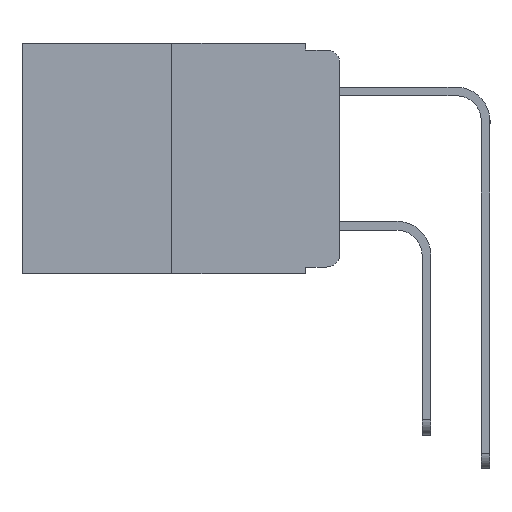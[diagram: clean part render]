
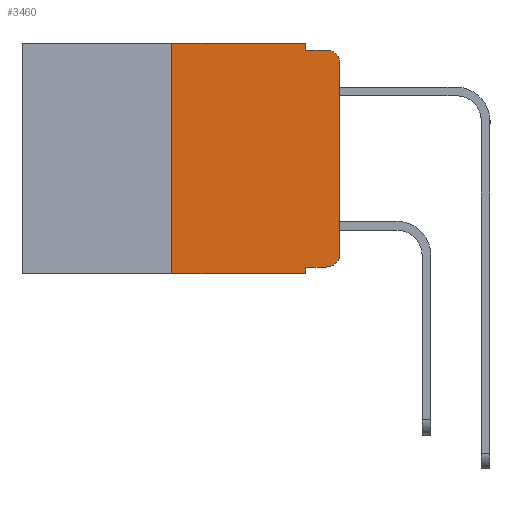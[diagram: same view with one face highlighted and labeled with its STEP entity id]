
A CAD part, left-side view. The second image highlights one B-rep face of the part: STEP entity #3460.
In plain terms, the highlighted planar face has unit normal (-1, 0, 0).
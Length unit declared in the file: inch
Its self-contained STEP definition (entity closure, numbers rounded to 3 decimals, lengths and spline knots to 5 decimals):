
#546 = VERTEX_POINT ( 'NONE', #12753 ) ;
#858 = CARTESIAN_POINT ( 'NONE',  ( 0., 0.02, -0.01 ) ) ;
#982 = ORIENTED_EDGE ( 'NONE', *, *, #9018, .F. ) ;
#1259 = VERTEX_POINT ( 'NONE', #13087 ) ;
#1698 = VERTEX_POINT ( 'NONE', #11523 ) ;
#2021 = PLANE ( 'NONE',  #4826 ) ;
#2198 = VERTEX_POINT ( 'NONE', #6630 ) ;
#2219 = DIRECTION ( 'NONE',  ( -1., 0., 0. ) ) ;
#2430 = VECTOR ( 'NONE', #13851, 39.37008 ) ;
#2683 = DIRECTION ( 'NONE',  ( 0., 0., 1. ) ) ;
#2816 = LINE ( 'NONE', #3233, #8758 ) ;
#3087 = CARTESIAN_POINT ( 'NONE',  ( 0., 0.473, 0. ) ) ;
#3233 = CARTESIAN_POINT ( 'NONE',  ( 0., 0.051, 0. ) ) ;
#3365 = CARTESIAN_POINT ( 'NONE',  ( 0., 0.051, 0. ) ) ;
#3460 = ADVANCED_FACE ( 'NONE', ( #4132 ), #2021, .F. ) ;
#3507 = VERTEX_POINT ( 'NONE', #858 ) ;
#3529 = VERTEX_POINT ( 'NONE', #14933 ) ;
#4132 = FACE_OUTER_BOUND ( 'NONE', #9407, .T. ) ;
#4143 = CIRCLE ( 'NONE', #9887, 0.02 ) ;
#4309 = DIRECTION ( 'NONE',  ( 0., -1., 0. ) ) ;
#4321 = VECTOR ( 'NONE', #9807, 39.37008 ) ;
#4395 = CARTESIAN_POINT ( 'NONE',  ( 0., 0.473, -0.343 ) ) ;
#4448 = DIRECTION ( 'NONE',  ( 1., 0., 0. ) ) ;
#4803 = EDGE_CURVE ( 'NONE', #1698, #1259, #10125, .T. ) ;
#4826 = AXIS2_PLACEMENT_3D ( 'NONE', #11409, #4448, #12557 ) ;
#5073 = CARTESIAN_POINT ( 'NONE',  ( 0., 0., 0. ) ) ;
#5165 = LINE ( 'NONE', #7351, #14039 ) ;
#5245 = ORIENTED_EDGE ( 'NONE', *, *, #7801, .T. ) ;
#5293 = DIRECTION ( 'NONE',  ( -1., 0., 0. ) ) ;
#5328 = ORIENTED_EDGE ( 'NONE', *, *, #4803, .F. ) ;
#5594 = VERTEX_POINT ( 'NONE', #12697 ) ;
#5635 = CARTESIAN_POINT ( 'NONE',  ( 0., 0.051, -0.01 ) ) ;
#6004 = ORIENTED_EDGE ( 'NONE', *, *, #7669, .F. ) ;
#6391 = CIRCLE ( 'NONE', #9435, 0.02 ) ;
#6630 = CARTESIAN_POINT ( 'NONE',  ( 0., 0.051, -0.333 ) ) ;
#6876 = ORIENTED_EDGE ( 'NONE', *, *, #14303, .F. ) ;
#6917 = VERTEX_POINT ( 'NONE', #13017 ) ;
#6990 = VECTOR ( 'NONE', #9794, 39.37008 ) ;
#7351 = CARTESIAN_POINT ( 'NONE',  ( 0., 0.25, 0. ) ) ;
#7669 = EDGE_CURVE ( 'NONE', #1259, #12660, #2816, .T. ) ;
#7801 = EDGE_CURVE ( 'NONE', #6917, #3529, #4143, .T. ) ;
#7950 = DIRECTION ( 'NONE',  ( 0., 0., -1. ) ) ;
#8338 = LINE ( 'NONE', #5635, #9075 ) ;
#8619 = CARTESIAN_POINT ( 'NONE',  ( 0., 0.051, -0.333 ) ) ;
#8758 = VECTOR ( 'NONE', #7950, 39.37008 ) ;
#8956 = VECTOR ( 'NONE', #10283, 39.37008 ) ;
#9018 = EDGE_CURVE ( 'NONE', #12660, #3507, #8338, .T. ) ;
#9051 = ORIENTED_EDGE ( 'NONE', *, *, #10479, .F. ) ;
#9075 = VECTOR ( 'NONE', #11428, 39.37008 ) ;
#9323 = CARTESIAN_POINT ( 'NONE',  ( 0., 0.02, -0.313 ) ) ;
#9367 = VERTEX_POINT ( 'NONE', #14521 ) ;
#9407 = EDGE_LOOP ( 'NONE', ( #10090, #10261, #982, #6004, #5328, #9051, #12597, #6876, #12274, #5245 ) ) ;
#9435 = AXIS2_PLACEMENT_3D ( 'NONE', #12228, #5293, #13392 ) ;
#9794 = DIRECTION ( 'NONE',  ( 0., -1., 0. ) ) ;
#9807 = DIRECTION ( 'NONE',  ( 0., 0., 1. ) ) ;
#9887 = AXIS2_PLACEMENT_3D ( 'NONE', #9323, #2219, #10470 ) ;
#10090 = ORIENTED_EDGE ( 'NONE', *, *, #14594, .T. ) ;
#10125 = LINE ( 'NONE', #3087, #12778 ) ;
#10261 = ORIENTED_EDGE ( 'NONE', *, *, #12276, .T. ) ;
#10283 = DIRECTION ( 'NONE',  ( 0., -1., 0. ) ) ;
#10470 = DIRECTION ( 'NONE',  ( 0., 0., -1. ) ) ;
#10479 = EDGE_CURVE ( 'NONE', #5594, #1698, #5165, .T. ) ;
#10522 = LINE ( 'NONE', #5073, #4321 ) ;
#10772 = EDGE_CURVE ( 'NONE', #2198, #6917, #13124, .T. ) ;
#11409 = CARTESIAN_POINT ( 'NONE',  ( 0., 0.473, 0. ) ) ;
#11428 = DIRECTION ( 'NONE',  ( 0., -1., 0. ) ) ;
#11523 = CARTESIAN_POINT ( 'NONE',  ( 0., 0.25, 0. ) ) ;
#11919 = CARTESIAN_POINT ( 'NONE',  ( 0., 0.051, -0.01 ) ) ;
#12228 = CARTESIAN_POINT ( 'NONE',  ( 0., 0.02, -0.03 ) ) ;
#12274 = ORIENTED_EDGE ( 'NONE', *, *, #10772, .T. ) ;
#12276 = EDGE_CURVE ( 'NONE', #546, #3507, #6391, .T. ) ;
#12557 = DIRECTION ( 'NONE',  ( 0., 0., -1. ) ) ;
#12597 = ORIENTED_EDGE ( 'NONE', *, *, #13621, .T. ) ;
#12660 = VERTEX_POINT ( 'NONE', #11919 ) ;
#12697 = CARTESIAN_POINT ( 'NONE',  ( 0., 0.25, -0.343 ) ) ;
#12753 = CARTESIAN_POINT ( 'NONE',  ( 0., 0., -0.03 ) ) ;
#12778 = VECTOR ( 'NONE', #4309, 39.37008 ) ;
#13017 = CARTESIAN_POINT ( 'NONE',  ( 0., 0.02, -0.333 ) ) ;
#13087 = CARTESIAN_POINT ( 'NONE',  ( 0., 0.051, 0. ) ) ;
#13124 = LINE ( 'NONE', #8619, #6990 ) ;
#13392 = DIRECTION ( 'NONE',  ( 0., 0., -1. ) ) ;
#13621 = EDGE_CURVE ( 'NONE', #5594, #9367, #14996, .T. ) ;
#13851 = DIRECTION ( 'NONE',  ( 0., 0., -1. ) ) ;
#14039 = VECTOR ( 'NONE', #2683, 39.37008 ) ;
#14303 = EDGE_CURVE ( 'NONE', #2198, #9367, #14810, .T. ) ;
#14521 = CARTESIAN_POINT ( 'NONE',  ( 0., 0.051, -0.343 ) ) ;
#14594 = EDGE_CURVE ( 'NONE', #3529, #546, #10522, .T. ) ;
#14810 = LINE ( 'NONE', #3365, #2430 ) ;
#14933 = CARTESIAN_POINT ( 'NONE',  ( 0., 0., -0.313 ) ) ;
#14996 = LINE ( 'NONE', #4395, #8956 ) ;
